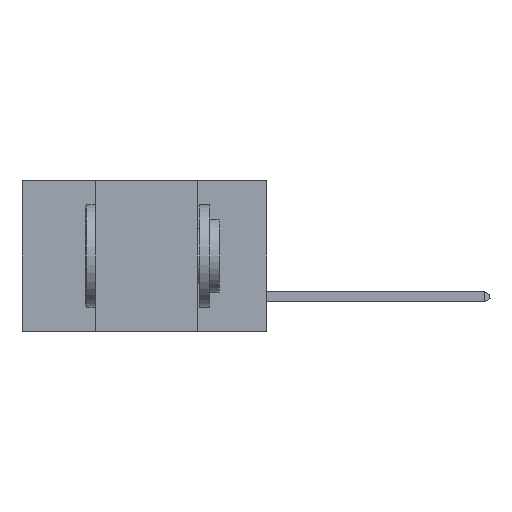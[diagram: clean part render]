
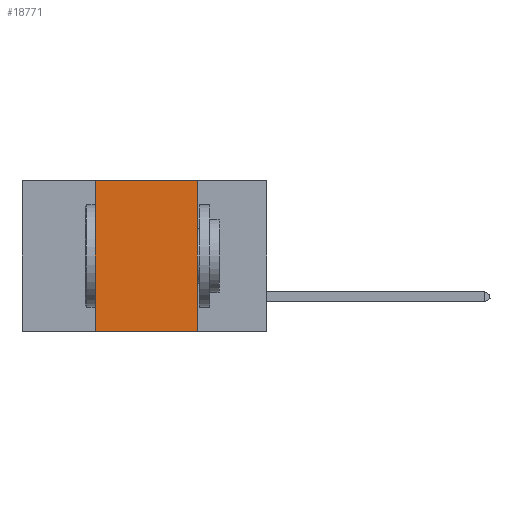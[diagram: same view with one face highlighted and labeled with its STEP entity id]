
A CAD part, left-side view. The second image highlights one B-rep face of the part: STEP entity #18771.
In plain terms, the highlighted planar face has unit normal (-1, 0, 0).
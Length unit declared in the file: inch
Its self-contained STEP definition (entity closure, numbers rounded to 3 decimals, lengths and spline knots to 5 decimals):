
#872 = DIRECTION ( 'NONE',  ( 1., 0., 0. ) ) ;
#2463 = CARTESIAN_POINT ( 'NONE',  ( 0., 0.6, 0. ) ) ;
#2534 = FACE_OUTER_BOUND ( 'NONE', #15405, .T. ) ;
#2906 = EDGE_CURVE ( 'NONE', #5645, #9522, #12045, .T. ) ;
#3026 = AXIS2_PLACEMENT_3D ( 'NONE', #21103, #872, #16131 ) ;
#3431 = ORIENTED_EDGE ( 'NONE', *, *, #2906, .F. ) ;
#4143 = DIRECTION ( 'NONE',  ( 0., -1., 0. ) ) ;
#4436 = CARTESIAN_POINT ( 'NONE',  ( 0., 0.17, -0.37 ) ) ;
#4485 = ORIENTED_EDGE ( 'NONE', *, *, #12426, .F. ) ;
#4490 = CARTESIAN_POINT ( 'NONE',  ( 0., 0.17, 0. ) ) ;
#5645 = VERTEX_POINT ( 'NONE', #8068 ) ;
#6448 = VECTOR ( 'NONE', #21207, 39.37008 ) ;
#6451 = CARTESIAN_POINT ( 'NONE',  ( 0., 0.42, -0.37 ) ) ;
#7567 = CARTESIAN_POINT ( 'NONE',  ( 0., 0.6, -0.37 ) ) ;
#7609 = PLANE ( 'NONE',  #3026 ) ;
#7866 = VECTOR ( 'NONE', #18057, 39.37008 ) ;
#8068 = CARTESIAN_POINT ( 'NONE',  ( 0., 0.42, 0. ) ) ;
#9522 = VERTEX_POINT ( 'NONE', #4490 ) ;
#10117 = VERTEX_POINT ( 'NONE', #6451 ) ;
#10134 = LINE ( 'NONE', #7567, #6448 ) ;
#12045 = LINE ( 'NONE', #2463, #14724 ) ;
#12426 = EDGE_CURVE ( 'NONE', #10117, #5645, #20401, .T. ) ;
#13051 = CARTESIAN_POINT ( 'NONE',  ( 0., 0.17, 0. ) ) ;
#14373 = VECTOR ( 'NONE', #17818, 39.37008 ) ;
#14724 = VECTOR ( 'NONE', #4143, 39.37008 ) ;
#15405 = EDGE_LOOP ( 'NONE', ( #20578, #3431, #4485, #19879 ) ) ;
#15622 = EDGE_CURVE ( 'NONE', #9522, #21713, #16855, .T. ) ;
#16015 = CARTESIAN_POINT ( 'NONE',  ( 0., 0.42, 0. ) ) ;
#16131 = DIRECTION ( 'NONE',  ( 0., 0., -1. ) ) ;
#16855 = LINE ( 'NONE', #13051, #7866 ) ;
#17818 = DIRECTION ( 'NONE',  ( 0., 0., 1. ) ) ;
#18057 = DIRECTION ( 'NONE',  ( 0., 0., -1. ) ) ;
#18771 = ADVANCED_FACE ( 'NONE', ( #2534 ), #7609, .F. ) ;
#19879 = ORIENTED_EDGE ( 'NONE', *, *, #20277, .T. ) ;
#20277 = EDGE_CURVE ( 'NONE', #10117, #21713, #10134, .T. ) ;
#20401 = LINE ( 'NONE', #16015, #14373 ) ;
#20578 = ORIENTED_EDGE ( 'NONE', *, *, #15622, .F. ) ;
#21103 = CARTESIAN_POINT ( 'NONE',  ( 0., 0.6, 0. ) ) ;
#21207 = DIRECTION ( 'NONE',  ( 0., -1., 0. ) ) ;
#21713 = VERTEX_POINT ( 'NONE', #4436 ) ;
